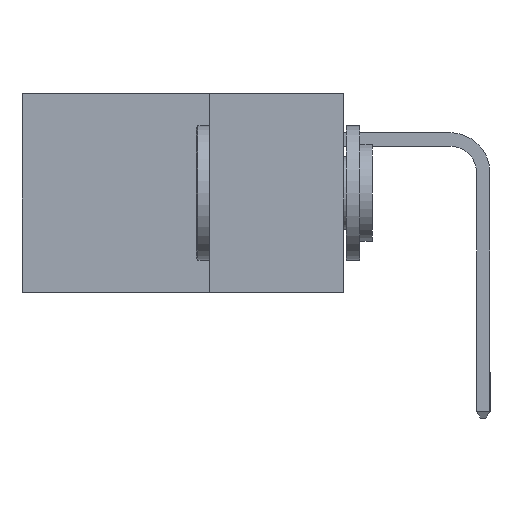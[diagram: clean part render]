
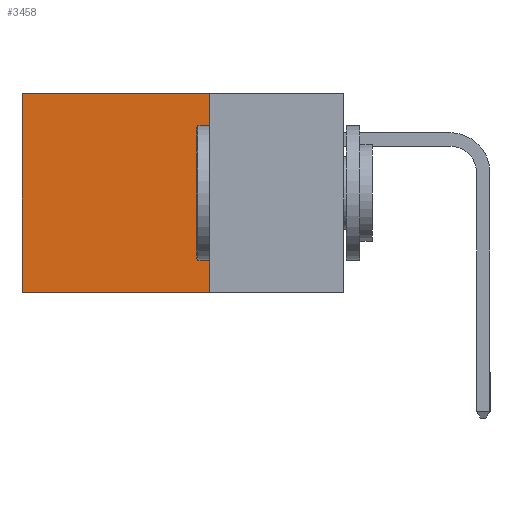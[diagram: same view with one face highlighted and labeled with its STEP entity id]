
A CAD part, left-side view. The second image highlights one B-rep face of the part: STEP entity #3458.
In plain terms, the highlighted planar face has unit normal (-1, 0, 0).
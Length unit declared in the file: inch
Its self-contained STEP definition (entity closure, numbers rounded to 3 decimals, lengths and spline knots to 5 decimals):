
#75 = CARTESIAN_POINT ( 'NONE',  ( 0.2615, 0.25, -0.37 ) ) ;
#346 = DIRECTION ( 'NONE',  ( 1., 0., 0. ) ) ;
#473 = DIRECTION ( 'NONE',  ( 0., 1., 0. ) ) ;
#569 = VECTOR ( 'NONE', #10566, 39.37008 ) ;
#667 = DIRECTION ( 'NONE',  ( 0., 0., -1. ) ) ;
#951 = LINE ( 'NONE', #13967, #3634 ) ;
#1643 = LINE ( 'NONE', #6384, #4563 ) ;
#3356 = DIRECTION ( 'NONE',  ( 0., 1., 0. ) ) ;
#3458 = ADVANCED_FACE ( 'NONE', ( #8873 ), #14782, .F. ) ;
#3634 = VECTOR ( 'NONE', #3356, 39.37008 ) ;
#3738 = LINE ( 'NONE', #75, #569 ) ;
#4059 = DIRECTION ( 'NONE',  ( 0., 0., -1. ) ) ;
#4327 = ORIENTED_EDGE ( 'NONE', *, *, #10403, .F. ) ;
#4563 = VECTOR ( 'NONE', #473, 39.37008 ) ;
#6030 = ORIENTED_EDGE ( 'NONE', *, *, #12719, .T. ) ;
#6384 = CARTESIAN_POINT ( 'NONE',  ( 0.2615, 0.25, -0.37 ) ) ;
#6742 = VERTEX_POINT ( 'NONE', #9132 ) ;
#6816 = LINE ( 'NONE', #6895, #9748 ) ;
#6895 = CARTESIAN_POINT ( 'NONE',  ( 0.2615, 0.6, -0.37 ) ) ;
#7487 = VERTEX_POINT ( 'NONE', #7547 ) ;
#7547 = CARTESIAN_POINT ( 'NONE',  ( 0.2615, 0.25, -0.37 ) ) ;
#7596 = ORIENTED_EDGE ( 'NONE', *, *, #11851, .F. ) ;
#7606 = AXIS2_PLACEMENT_3D ( 'NONE', #14865, #346, #4059 ) ;
#8788 = EDGE_LOOP ( 'NONE', ( #6030, #7596, #4327, #12963 ) ) ;
#8873 = FACE_OUTER_BOUND ( 'NONE', #8788, .T. ) ;
#9132 = CARTESIAN_POINT ( 'NONE',  ( 0.2615, 0.6, 0. ) ) ;
#9216 = EDGE_CURVE ( 'NONE', #12357, #6742, #951, .T. ) ;
#9748 = VECTOR ( 'NONE', #667, 39.37008 ) ;
#10403 = EDGE_CURVE ( 'NONE', #12357, #7487, #3738, .T. ) ;
#10566 = DIRECTION ( 'NONE',  ( 0., 0., -1. ) ) ;
#11851 = EDGE_CURVE ( 'NONE', #7487, #12934, #1643, .T. ) ;
#12357 = VERTEX_POINT ( 'NONE', #14963 ) ;
#12719 = EDGE_CURVE ( 'NONE', #6742, #12934, #6816, .T. ) ;
#12934 = VERTEX_POINT ( 'NONE', #13158 ) ;
#12963 = ORIENTED_EDGE ( 'NONE', *, *, #9216, .T. ) ;
#13158 = CARTESIAN_POINT ( 'NONE',  ( 0.2615, 0.6, -0.37 ) ) ;
#13967 = CARTESIAN_POINT ( 'NONE',  ( 0.2615, 0.25, 0. ) ) ;
#14782 = PLANE ( 'NONE',  #7606 ) ;
#14865 = CARTESIAN_POINT ( 'NONE',  ( 0.2615, 0.25, -0.37 ) ) ;
#14963 = CARTESIAN_POINT ( 'NONE',  ( 0.2615, 0.25, 0. ) ) ;
